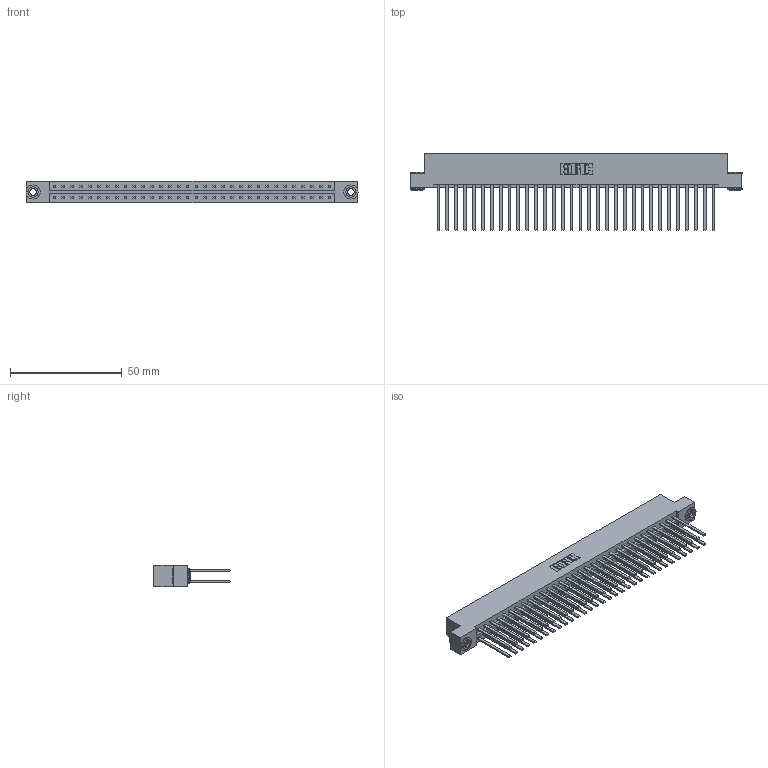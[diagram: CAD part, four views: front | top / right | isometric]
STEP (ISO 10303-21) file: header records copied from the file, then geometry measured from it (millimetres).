
FILE_DESCRIPTION (( 'STEP AP203' ), '1' );
FILE_NAME ('833-064-544-203.STEP', '2020-06-05T07:31:12', ( '' ), ( '' ), 'SwSTEP 2.0', 'SolidWorks 2020', '' );
FILE_SCHEMA (( 'CONFIG_CONTROL_DESIGN' ));
Length unit declared in the file: inch
Products named in the file (4): 345-250-002_345-250-002-102; 833 Part_Flush - .156 Dia - TH; 833-064-544-203; 345-292-001_345-293-144
Assembly tree (67 placements, depth 2):
  833-064-544-203
    833 Part_Flush - .156 Dia - TH
    345-292-001_345-293-144  x64
    345-250-002_345-250-002-102  x2
Bounding box: 148.34 x 34.3 x 9.4 mm (x, y, z)
Volume: 15967.3 mm3; surface area: 21879.4 mm2
Topology: 67 solids, 67 shells, 3096 faces, 9155 edges, 6014 vertices
Faces by surface type: plane 2128, cylinder 960, cone 8
Entity records: 22346 total; most frequent: CARTESIAN_POINT 3689, ORIENTED_EDGE 3618, DIRECTION 3199, EDGE_CURVE 1809, VECTOR 1661, LINE 1661, VERTEX_POINT 1202, AXIS2_PLACEMENT_3D 769
